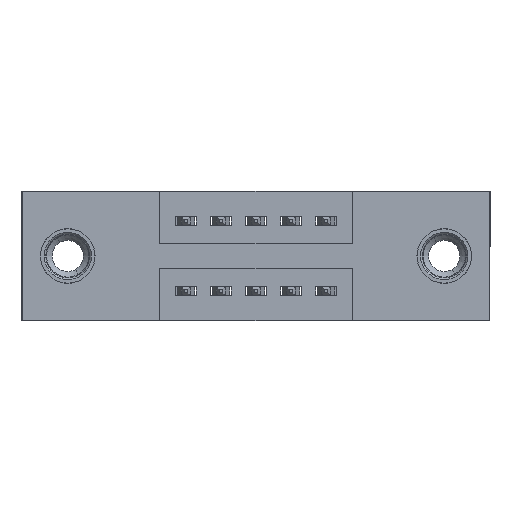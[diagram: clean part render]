
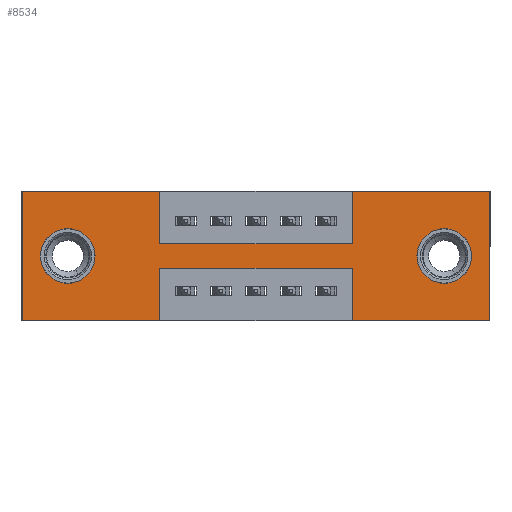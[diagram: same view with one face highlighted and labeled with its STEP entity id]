
A CAD part, front view. The second image highlights one B-rep face of the part: STEP entity #8534.
In plain terms, the highlighted planar face has unit normal (0, -1, 0).
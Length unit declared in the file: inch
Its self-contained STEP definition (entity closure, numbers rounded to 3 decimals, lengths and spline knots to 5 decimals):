
#23 = CARTESIAN_POINT ( 'NONE',  ( 0.3925, 0., -0.22 ) ) ;
#97 = DIRECTION ( 'NONE',  ( 0., 0., 1. ) ) ;
#111 = VERTEX_POINT ( 'NONE', #10083 ) ;
#275 = CARTESIAN_POINT ( 'NONE',  ( 1.205, 0., -0.107 ) ) ;
#337 = DIRECTION ( 'NONE',  ( 0., 0., -1. ) ) ;
#372 = VERTEX_POINT ( 'NONE', #4202 ) ;
#377 = CARTESIAN_POINT ( 'NONE',  ( 0.9425, 0., 0. ) ) ;
#413 = CARTESIAN_POINT ( 'NONE',  ( 0.3925, 0., -0.37 ) ) ;
#425 = ORIENTED_EDGE ( 'NONE', *, *, #9686, .T. ) ;
#438 = DIRECTION ( 'NONE',  ( 0., 1., 0. ) ) ;
#547 = VECTOR ( 'NONE', #4108, 39.37008 ) ;
#607 = VERTEX_POINT ( 'NONE', #5448 ) ;
#826 = CARTESIAN_POINT ( 'NONE',  ( 0., 0., -0.37 ) ) ;
#903 = CARTESIAN_POINT ( 'NONE',  ( 0.3925, 0., 0. ) ) ;
#1032 = ORIENTED_EDGE ( 'NONE', *, *, #6242, .F. ) ;
#1428 = VECTOR ( 'NONE', #5306, 39.37008 ) ;
#1683 = CARTESIAN_POINT ( 'NONE',  ( 0.3925, 0., 0. ) ) ;
#1960 = VERTEX_POINT ( 'NONE', #377 ) ;
#2120 = DIRECTION ( 'NONE',  ( 1., 0., 0. ) ) ;
#2146 = EDGE_CURVE ( 'NONE', #111, #7626, #9634, .T. ) ;
#2170 = CARTESIAN_POINT ( 'NONE',  ( 0., 0., 0. ) ) ;
#2182 = VERTEX_POINT ( 'NONE', #3406 ) ;
#2225 = VECTOR ( 'NONE', #4363, 39.37008 ) ;
#2256 = ORIENTED_EDGE ( 'NONE', *, *, #7274, .T. ) ;
#2275 = VERTEX_POINT ( 'NONE', #2910 ) ;
#2521 = CARTESIAN_POINT ( 'NONE',  ( 0.13, 0., -0.185 ) ) ;
#2614 = ORIENTED_EDGE ( 'NONE', *, *, #2146, .F. ) ;
#2632 = VECTOR ( 'NONE', #2120, 39.37008 ) ;
#2782 = VECTOR ( 'NONE', #6903, 39.37008 ) ;
#2793 = VECTOR ( 'NONE', #2901, 39.37008 ) ;
#2806 = CARTESIAN_POINT ( 'NONE',  ( 0., 0., 0. ) ) ;
#2901 = DIRECTION ( 'NONE',  ( -1., 0., 0. ) ) ;
#2910 = CARTESIAN_POINT ( 'NONE',  ( 0.3925, 0., -0.37 ) ) ;
#2957 = EDGE_CURVE ( 'NONE', #4620, #372, #5430, .T. ) ;
#2980 = CIRCLE ( 'NONE', #4522, 0.078 ) ;
#3009 = VERTEX_POINT ( 'NONE', #23 ) ;
#3094 = CARTESIAN_POINT ( 'NONE',  ( 0.9425, 0., -0.22 ) ) ;
#3110 = DIRECTION ( 'NONE',  ( 0., 0., 1. ) ) ;
#3186 = CARTESIAN_POINT ( 'NONE',  ( 0., 0., -0.37 ) ) ;
#3216 = AXIS2_PLACEMENT_3D ( 'NONE', #2521, #8280, #3411 ) ;
#3230 = LINE ( 'NONE', #903, #9478 ) ;
#3286 = CARTESIAN_POINT ( 'NONE',  ( 1.335, 0., 0. ) ) ;
#3378 = ORIENTED_EDGE ( 'NONE', *, *, #4192, .F. ) ;
#3406 = CARTESIAN_POINT ( 'NONE',  ( 0.13, 0., -0.107 ) ) ;
#3411 = DIRECTION ( 'NONE',  ( 0., 0., 1. ) ) ;
#3471 = VERTEX_POINT ( 'NONE', #3186 ) ;
#3551 = LINE ( 'NONE', #7985, #5465 ) ;
#3666 = DIRECTION ( 'NONE',  ( 0., -1., 0. ) ) ;
#3889 = CARTESIAN_POINT ( 'NONE',  ( 0.9425, 0., -0.37 ) ) ;
#3899 = ORIENTED_EDGE ( 'NONE', *, *, #5837, .F. ) ;
#3917 = CARTESIAN_POINT ( 'NONE',  ( 0.3925, 0., -0.15 ) ) ;
#4067 = DIRECTION ( 'NONE',  ( -1., 0., 0. ) ) ;
#4108 = DIRECTION ( 'NONE',  ( 0., 0., 1. ) ) ;
#4192 = EDGE_CURVE ( 'NONE', #3009, #2275, #8050, .T. ) ;
#4202 = CARTESIAN_POINT ( 'NONE',  ( 1.205, 0., -0.263 ) ) ;
#4363 = DIRECTION ( 'NONE',  ( 1., 0., 0. ) ) ;
#4375 = LINE ( 'NONE', #2170, #2632 ) ;
#4443 = AXIS2_PLACEMENT_3D ( 'NONE', #10020, #5173, #10856 ) ;
#4482 = ORIENTED_EDGE ( 'NONE', *, *, #8028, .T. ) ;
#4494 = EDGE_CURVE ( 'NONE', #1960, #10247, #9095, .T. ) ;
#4508 = CARTESIAN_POINT ( 'NONE',  ( 1.205, 0., -0.185 ) ) ;
#4509 = CARTESIAN_POINT ( 'NONE',  ( 0.13, 0., -0.263 ) ) ;
#4522 = AXIS2_PLACEMENT_3D ( 'NONE', #10349, #5505, #97 ) ;
#4620 = VERTEX_POINT ( 'NONE', #275 ) ;
#4735 = LINE ( 'NONE', #9442, #8791 ) ;
#5038 = LINE ( 'NONE', #8621, #2793 ) ;
#5173 = DIRECTION ( 'NONE',  ( 0., 1., 0. ) ) ;
#5196 = EDGE_CURVE ( 'NONE', #607, #5481, #4375, .T. ) ;
#5306 = DIRECTION ( 'NONE',  ( -1., 0., 0. ) ) ;
#5349 = ORIENTED_EDGE ( 'NONE', *, *, #9955, .F. ) ;
#5430 = CIRCLE ( 'NONE', #6369, 0.078 ) ;
#5448 = CARTESIAN_POINT ( 'NONE',  ( 0., 0., 0. ) ) ;
#5465 = VECTOR ( 'NONE', #3110, 39.37008 ) ;
#5481 = VERTEX_POINT ( 'NONE', #1683 ) ;
#5505 = DIRECTION ( 'NONE',  ( 0., 1., 0. ) ) ;
#5647 = CARTESIAN_POINT ( 'NONE',  ( 0., 0., -0.37 ) ) ;
#5837 = EDGE_CURVE ( 'NONE', #7287, #111, #10713, .T. ) ;
#5898 = VECTOR ( 'NONE', #6562, 39.37008 ) ;
#6025 = LINE ( 'NONE', #9345, #10339 ) ;
#6242 = EDGE_CURVE ( 'NONE', #9877, #1960, #4735, .T. ) ;
#6369 = AXIS2_PLACEMENT_3D ( 'NONE', #4508, #438, #337 ) ;
#6562 = DIRECTION ( 'NONE',  ( 0., 0., -1. ) ) ;
#6687 = LINE ( 'NONE', #8422, #2225 ) ;
#6760 = ORIENTED_EDGE ( 'NONE', *, *, #10534, .F. ) ;
#6903 = DIRECTION ( 'NONE',  ( 1., 0., 0. ) ) ;
#7013 = EDGE_CURVE ( 'NONE', #3471, #607, #3551, .T. ) ;
#7222 = CIRCLE ( 'NONE', #4443, 0.078 ) ;
#7244 = ORIENTED_EDGE ( 'NONE', *, *, #2957, .T. ) ;
#7274 = EDGE_CURVE ( 'NONE', #372, #4620, #7222, .T. ) ;
#7287 = VERTEX_POINT ( 'NONE', #8381 ) ;
#7576 = VERTEX_POINT ( 'NONE', #3917 ) ;
#7626 = VERTEX_POINT ( 'NONE', #3094 ) ;
#7736 = CARTESIAN_POINT ( 'NONE',  ( 0.3925, 0., -0.22 ) ) ;
#7784 = DIRECTION ( 'NONE',  ( 0., 0., -1. ) ) ;
#7948 = FACE_BOUND ( 'NONE', #8974, .T. ) ;
#7985 = CARTESIAN_POINT ( 'NONE',  ( 0., 0., 0. ) ) ;
#8028 = EDGE_CURVE ( 'NONE', #2182, #8551, #2980, .T. ) ;
#8050 = LINE ( 'NONE', #413, #5898 ) ;
#8280 = DIRECTION ( 'NONE',  ( 0., 1., 0. ) ) ;
#8381 = CARTESIAN_POINT ( 'NONE',  ( 1.335, 0., -0.37 ) ) ;
#8422 = CARTESIAN_POINT ( 'NONE',  ( 0.3925, 0., -0.15 ) ) ;
#8471 = ORIENTED_EDGE ( 'NONE', *, *, #5196, .F. ) ;
#8534 = ADVANCED_FACE ( 'NONE', ( #7948, #10116, #10369 ), #9332, .T. ) ;
#8536 = VECTOR ( 'NONE', #4067, 39.37008 ) ;
#8551 = VERTEX_POINT ( 'NONE', #4509 ) ;
#8617 = DIRECTION ( 'NONE',  ( 0., 0., 1. ) ) ;
#8621 = CARTESIAN_POINT ( 'NONE',  ( 0., 0., -0.37 ) ) ;
#8791 = VECTOR ( 'NONE', #8617, 39.37008 ) ;
#8974 = EDGE_LOOP ( 'NONE', ( #7244, #2256 ) ) ;
#8998 = EDGE_LOOP ( 'NONE', ( #4482, #425 ) ) ;
#9095 = LINE ( 'NONE', #2806, #2782 ) ;
#9223 = AXIS2_PLACEMENT_3D ( 'NONE', #826, #3666, #9365 ) ;
#9237 = ORIENTED_EDGE ( 'NONE', *, *, #9806, .F. ) ;
#9332 = PLANE ( 'NONE',  #9223 ) ;
#9345 = CARTESIAN_POINT ( 'NONE',  ( 1.335, 0., 0. ) ) ;
#9365 = DIRECTION ( 'NONE',  ( 0., 0., -1. ) ) ;
#9442 = CARTESIAN_POINT ( 'NONE',  ( 0.9425, 0., 0. ) ) ;
#9478 = VECTOR ( 'NONE', #7784, 39.37008 ) ;
#9634 = LINE ( 'NONE', #3889, #547 ) ;
#9686 = EDGE_CURVE ( 'NONE', #8551, #2182, #9875, .T. ) ;
#9755 = ORIENTED_EDGE ( 'NONE', *, *, #7013, .F. ) ;
#9806 = EDGE_CURVE ( 'NONE', #7576, #9877, #6687, .T. ) ;
#9875 = CIRCLE ( 'NONE', #3216, 0.078 ) ;
#9877 = VERTEX_POINT ( 'NONE', #10971 ) ;
#9941 = ORIENTED_EDGE ( 'NONE', *, *, #10616, .F. ) ;
#9955 = EDGE_CURVE ( 'NONE', #5481, #7576, #3230, .T. ) ;
#10020 = CARTESIAN_POINT ( 'NONE',  ( 1.205, 0., -0.185 ) ) ;
#10083 = CARTESIAN_POINT ( 'NONE',  ( 0.9425, 0., -0.37 ) ) ;
#10087 = LINE ( 'NONE', #7736, #1428 ) ;
#10116 = FACE_BOUND ( 'NONE', #8998, .T. ) ;
#10142 = DIRECTION ( 'NONE',  ( 0., 0., -1. ) ) ;
#10247 = VERTEX_POINT ( 'NONE', #3286 ) ;
#10339 = VECTOR ( 'NONE', #10142, 39.37008 ) ;
#10349 = CARTESIAN_POINT ( 'NONE',  ( 0.13, 0., -0.185 ) ) ;
#10369 = FACE_OUTER_BOUND ( 'NONE', #10904, .T. ) ;
#10499 = EDGE_CURVE ( 'NONE', #10247, #7287, #6025, .T. ) ;
#10534 = EDGE_CURVE ( 'NONE', #7626, #3009, #10087, .T. ) ;
#10616 = EDGE_CURVE ( 'NONE', #2275, #3471, #5038, .T. ) ;
#10713 = LINE ( 'NONE', #5647, #8536 ) ;
#10794 = ORIENTED_EDGE ( 'NONE', *, *, #4494, .F. ) ;
#10856 = DIRECTION ( 'NONE',  ( 0., 0., -1. ) ) ;
#10904 = EDGE_LOOP ( 'NONE', ( #3378, #6760, #2614, #3899, #11002, #10794, #1032, #9237, #5349, #8471, #9755, #9941 ) ) ;
#10971 = CARTESIAN_POINT ( 'NONE',  ( 0.9425, 0., -0.15 ) ) ;
#11002 = ORIENTED_EDGE ( 'NONE', *, *, #10499, .F. ) ;
